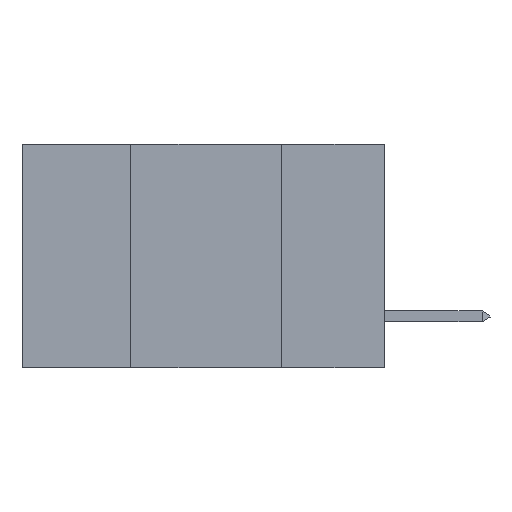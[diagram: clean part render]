
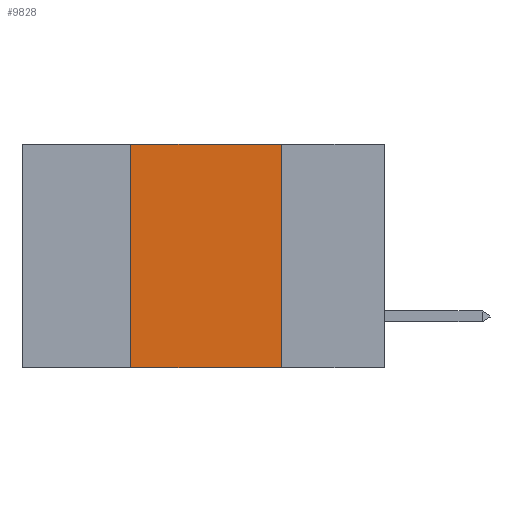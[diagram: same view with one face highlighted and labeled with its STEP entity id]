
A CAD part, left-side view. The second image highlights one B-rep face of the part: STEP entity #9828.
In plain terms, the highlighted planar face has unit normal (-1, 0, 0).
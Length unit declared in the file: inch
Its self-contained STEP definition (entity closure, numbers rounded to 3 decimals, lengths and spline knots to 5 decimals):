
#1112 = CARTESIAN_POINT ( 'NONE',  ( 0., 0.6, -0.37 ) ) ;
#2234 = CARTESIAN_POINT ( 'NONE',  ( 0., 0.6, 0. ) ) ;
#2251 = FACE_OUTER_BOUND ( 'NONE', #17452, .T. ) ;
#3041 = EDGE_CURVE ( 'NONE', #8180, #23844, #24778, .T. ) ;
#3400 = LINE ( 'NONE', #3485, #12830 ) ;
#3485 = CARTESIAN_POINT ( 'NONE',  ( 0., 0.17, 0. ) ) ;
#3688 = EDGE_CURVE ( 'NONE', #8180, #5786, #13694, .T. ) ;
#3735 = CARTESIAN_POINT ( 'NONE',  ( 0., 0.17, 0. ) ) ;
#3904 = PLANE ( 'NONE',  #16733 ) ;
#4369 = ORIENTED_EDGE ( 'NONE', *, *, #3041, .F. ) ;
#5638 = DIRECTION ( 'NONE',  ( 0., 0., -1. ) ) ;
#5786 = VERTEX_POINT ( 'NONE', #9380 ) ;
#6164 = CARTESIAN_POINT ( 'NONE',  ( 0., 0.42, 0. ) ) ;
#8180 = VERTEX_POINT ( 'NONE', #13079 ) ;
#9380 = CARTESIAN_POINT ( 'NONE',  ( 0., 0.17, -0.37 ) ) ;
#9828 = ADVANCED_FACE ( 'NONE', ( #2251 ), #3904, .F. ) ;
#10974 = EDGE_CURVE ( 'NONE', #23844, #25735, #21112, .T. ) ;
#12400 = DIRECTION ( 'NONE',  ( 0., 0., 1. ) ) ;
#12658 = ORIENTED_EDGE ( 'NONE', *, *, #10974, .F. ) ;
#12830 = VECTOR ( 'NONE', #21900, 39.37008 ) ;
#13079 = CARTESIAN_POINT ( 'NONE',  ( 0., 0.42, -0.37 ) ) ;
#13694 = LINE ( 'NONE', #1112, #24419 ) ;
#13742 = VECTOR ( 'NONE', #12400, 39.37008 ) ;
#14622 = EDGE_CURVE ( 'NONE', #25735, #5786, #3400, .T. ) ;
#16733 = AXIS2_PLACEMENT_3D ( 'NONE', #18035, #18404, #5638 ) ;
#16899 = ORIENTED_EDGE ( 'NONE', *, *, #14622, .F. ) ;
#17452 = EDGE_LOOP ( 'NONE', ( #16899, #12658, #4369, #19691 ) ) ;
#18035 = CARTESIAN_POINT ( 'NONE',  ( 0., 0.6, 0. ) ) ;
#18404 = DIRECTION ( 'NONE',  ( 1., 0., 0. ) ) ;
#19691 = ORIENTED_EDGE ( 'NONE', *, *, #3688, .T. ) ;
#20138 = VECTOR ( 'NONE', #25165, 39.37008 ) ;
#20698 = DIRECTION ( 'NONE',  ( 0., -1., 0. ) ) ;
#21112 = LINE ( 'NONE', #2234, #20138 ) ;
#21810 = CARTESIAN_POINT ( 'NONE',  ( 0., 0.42, 0. ) ) ;
#21900 = DIRECTION ( 'NONE',  ( 0., 0., -1. ) ) ;
#23844 = VERTEX_POINT ( 'NONE', #21810 ) ;
#24419 = VECTOR ( 'NONE', #20698, 39.37008 ) ;
#24778 = LINE ( 'NONE', #6164, #13742 ) ;
#25165 = DIRECTION ( 'NONE',  ( 0., -1., 0. ) ) ;
#25735 = VERTEX_POINT ( 'NONE', #3735 ) ;
